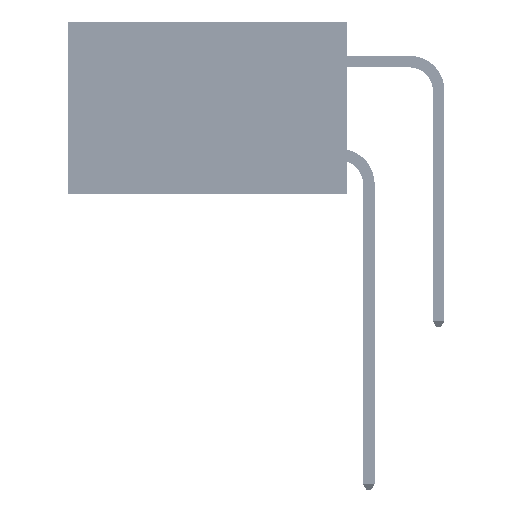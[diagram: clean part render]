
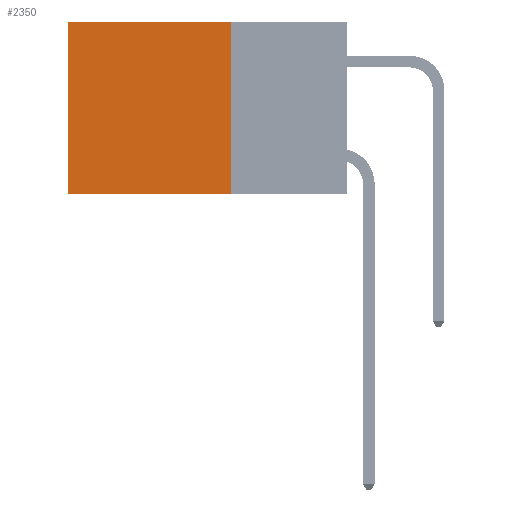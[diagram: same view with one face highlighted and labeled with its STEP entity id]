
A CAD part, left-side view. The second image highlights one B-rep face of the part: STEP entity #2350.
In plain terms, the highlighted planar face has unit normal (-1, 0, 0).
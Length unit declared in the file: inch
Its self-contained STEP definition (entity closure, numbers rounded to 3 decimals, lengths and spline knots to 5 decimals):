
#1650 = ORIENTED_EDGE ( 'NONE', *, *, #31492, .F. ) ;
#1721 = VERTEX_POINT ( 'NONE', #28163 ) ;
#2350 = ADVANCED_FACE ( 'NONE', ( #35239 ), #39377, .F. ) ;
#2930 = CARTESIAN_POINT ( 'NONE',  ( 0.2875, 0.6, 0. ) ) ;
#2984 = VERTEX_POINT ( 'NONE', #45124 ) ;
#5246 = CARTESIAN_POINT ( 'NONE',  ( 0.2875, 0.25, 0. ) ) ;
#5910 = CARTESIAN_POINT ( 'NONE',  ( 0.2875, 0.25, -0.37 ) ) ;
#6414 = DIRECTION ( 'NONE',  ( 1., 0., 0. ) ) ;
#7551 = AXIS2_PLACEMENT_3D ( 'NONE', #35990, #6414, #13795 ) ;
#11674 = EDGE_CURVE ( 'NONE', #39412, #2984, #26173, .T. ) ;
#12557 = VECTOR ( 'NONE', #46078, 39.37008 ) ;
#13069 = CARTESIAN_POINT ( 'NONE',  ( 0.2875, 0.6, 0. ) ) ;
#13795 = DIRECTION ( 'NONE',  ( 0., 0., -1. ) ) ;
#14079 = VECTOR ( 'NONE', #34907, 39.37008 ) ;
#14262 = DIRECTION ( 'NONE',  ( 0., 1., 0. ) ) ;
#15041 = ORIENTED_EDGE ( 'NONE', *, *, #11674, .T. ) ;
#19551 = VERTEX_POINT ( 'NONE', #28721 ) ;
#20700 = ORIENTED_EDGE ( 'NONE', *, *, #31663, .T. ) ;
#24188 = VECTOR ( 'NONE', #14262, 39.37008 ) ;
#26173 = LINE ( 'NONE', #13069, #14079 ) ;
#28163 = CARTESIAN_POINT ( 'NONE',  ( 0.2875, 0.25, 0. ) ) ;
#28721 = CARTESIAN_POINT ( 'NONE',  ( 0.2875, 0.25, -0.37 ) ) ;
#30527 = LINE ( 'NONE', #5910, #34506 ) ;
#31492 = EDGE_CURVE ( 'NONE', #19551, #2984, #30527, .T. ) ;
#31663 = EDGE_CURVE ( 'NONE', #1721, #39412, #39709, .T. ) ;
#34506 = VECTOR ( 'NONE', #35498, 39.37008 ) ;
#34866 = EDGE_CURVE ( 'NONE', #1721, #19551, #36132, .T. ) ;
#34907 = DIRECTION ( 'NONE',  ( 0., 0., -1. ) ) ;
#35239 = FACE_OUTER_BOUND ( 'NONE', #36905, .T. ) ;
#35498 = DIRECTION ( 'NONE',  ( 0., 1., 0. ) ) ;
#35990 = CARTESIAN_POINT ( 'NONE',  ( 0.2875, 0.25, 0. ) ) ;
#36132 = LINE ( 'NONE', #5246, #12557 ) ;
#36905 = EDGE_LOOP ( 'NONE', ( #15041, #1650, #42841, #20700 ) ) ;
#39377 = PLANE ( 'NONE',  #7551 ) ;
#39412 = VERTEX_POINT ( 'NONE', #2930 ) ;
#39709 = LINE ( 'NONE', #47083, #24188 ) ;
#42841 = ORIENTED_EDGE ( 'NONE', *, *, #34866, .F. ) ;
#45124 = CARTESIAN_POINT ( 'NONE',  ( 0.2875, 0.6, -0.37 ) ) ;
#46078 = DIRECTION ( 'NONE',  ( 0., 0., -1. ) ) ;
#47083 = CARTESIAN_POINT ( 'NONE',  ( 0.2875, 0.25, 0. ) ) ;
